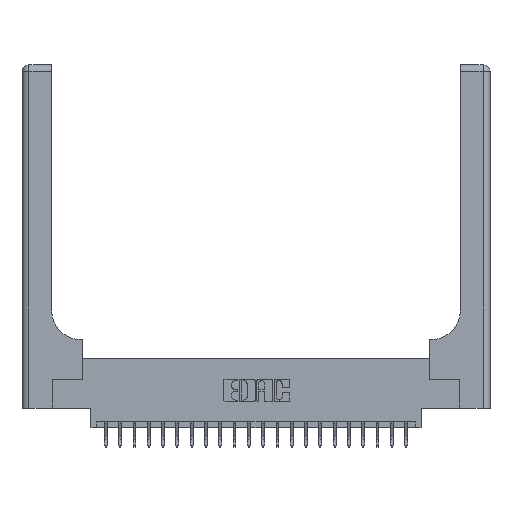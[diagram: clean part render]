
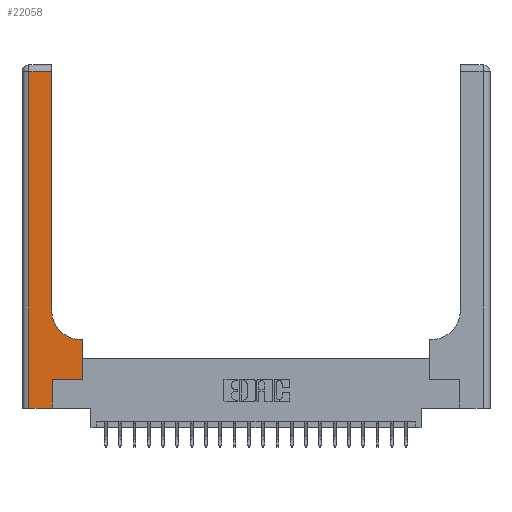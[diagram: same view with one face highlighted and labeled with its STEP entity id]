
A CAD part, top view. The second image highlights one B-rep face of the part: STEP entity #22058.
In plain terms, the highlighted planar face has unit normal (0, 0, 1).
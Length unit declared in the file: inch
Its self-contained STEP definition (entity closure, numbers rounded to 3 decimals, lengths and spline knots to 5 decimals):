
#354 = EDGE_CURVE ( 'NONE', #22687, #10060, #12485, .T. ) ;
#373 = DIRECTION ( 'NONE',  ( 0., 1., 0. ) ) ;
#702 = LINE ( 'NONE', #4646, #15385 ) ;
#1001 = VECTOR ( 'NONE', #373, 39.37008 ) ;
#1031 = VERTEX_POINT ( 'NONE', #20123 ) ;
#1869 = ORIENTED_EDGE ( 'NONE', *, *, #354, .T. ) ;
#2169 = FACE_OUTER_BOUND ( 'NONE', #19576, .T. ) ;
#2433 = AXIS2_PLACEMENT_3D ( 'NONE', #6753, #10251, #6408 ) ;
#2527 = CARTESIAN_POINT ( 'NONE',  ( 0.26, 0.85, 0.37 ) ) ;
#2699 = EDGE_CURVE ( 'NONE', #20403, #5717, #10989, .T. ) ;
#2760 = ORIENTED_EDGE ( 'NONE', *, *, #2699, .T. ) ;
#3105 = VECTOR ( 'NONE', #9244, 39.37008 ) ;
#3451 = DIRECTION ( 'NONE',  ( 0., 0., -1. ) ) ;
#3487 = CARTESIAN_POINT ( 'NONE',  ( 0.26, 0.6, 0.37 ) ) ;
#4061 = VERTEX_POINT ( 'NONE', #10677 ) ;
#4200 = VERTEX_POINT ( 'NONE', #21953 ) ;
#4477 = ORIENTED_EDGE ( 'NONE', *, *, #10024, .T. ) ;
#4501 = EDGE_CURVE ( 'NONE', #14902, #20403, #19275, .T. ) ;
#4569 = VERTEX_POINT ( 'NONE', #9562 ) ;
#4646 = CARTESIAN_POINT ( 'NONE',  ( 0.265, 0.25, 0.37 ) ) ;
#5717 = VERTEX_POINT ( 'NONE', #22329 ) ;
#5737 = AXIS2_PLACEMENT_3D ( 'NONE', #9171, #3451, #10915 ) ;
#6200 = ORIENTED_EDGE ( 'NONE', *, *, #15142, .T. ) ;
#6408 = DIRECTION ( 'NONE',  ( 1., 0., 0. ) ) ;
#6609 = CARTESIAN_POINT ( 'NONE',  ( 0.06, 0., 0.37 ) ) ;
#6746 = VECTOR ( 'NONE', #12349, 39.37008 ) ;
#6753 = CARTESIAN_POINT ( 'NONE',  ( 0.51, 0.85, 0.37 ) ) ;
#6793 = VECTOR ( 'NONE', #21531, 39.37008 ) ;
#6999 = CARTESIAN_POINT ( 'NONE',  ( 0., 2.94, 0.37 ) ) ;
#7068 = VECTOR ( 'NONE', #19384, 39.37008 ) ;
#7330 = LINE ( 'NONE', #14432, #6793 ) ;
#7454 = CARTESIAN_POINT ( 'NONE',  ( 0.265, 0., 0.37 ) ) ;
#7826 = DIRECTION ( 'NONE',  ( 1., 0., 0. ) ) ;
#7967 = CARTESIAN_POINT ( 'NONE',  ( 0.51, 0.6, 0.37 ) ) ;
#8855 = DIRECTION ( 'NONE',  ( -1., 0., 0. ) ) ;
#8887 = CARTESIAN_POINT ( 'NONE',  ( 0., 0., 0.37 ) ) ;
#9171 = CARTESIAN_POINT ( 'NONE',  ( 0., 3., 0.37 ) ) ;
#9244 = DIRECTION ( 'NONE',  ( 1., 0., 0. ) ) ;
#9562 = CARTESIAN_POINT ( 'NONE',  ( 0.26, 2.94, 0.37 ) ) ;
#10024 = EDGE_CURVE ( 'NONE', #4200, #1031, #7330, .T. ) ;
#10060 = VERTEX_POINT ( 'NONE', #2527 ) ;
#10251 = DIRECTION ( 'NONE',  ( 0., 0., -1. ) ) ;
#10677 = CARTESIAN_POINT ( 'NONE',  ( 0.265, 0.25, 0.37 ) ) ;
#10915 = DIRECTION ( 'NONE',  ( -1., 0., 0. ) ) ;
#10989 = LINE ( 'NONE', #8887, #3105 ) ;
#12276 = CARTESIAN_POINT ( 'NONE',  ( 0.06, 3., 0.37 ) ) ;
#12349 = DIRECTION ( 'NONE',  ( -1., 0., 0. ) ) ;
#12485 = CIRCLE ( 'NONE', #2433, 0.25 ) ;
#12688 = LINE ( 'NONE', #7454, #14801 ) ;
#13107 = ORIENTED_EDGE ( 'NONE', *, *, #4501, .T. ) ;
#13527 = ORIENTED_EDGE ( 'NONE', *, *, #17613, .T. ) ;
#14432 = CARTESIAN_POINT ( 'NONE',  ( 0.528, 0.25, 0.37 ) ) ;
#14550 = DIRECTION ( 'NONE',  ( 0., 1., 0. ) ) ;
#14801 = VECTOR ( 'NONE', #14550, 39.37008 ) ;
#14902 = VERTEX_POINT ( 'NONE', #15537 ) ;
#15142 = EDGE_CURVE ( 'NONE', #10060, #4569, #21587, .T. ) ;
#15158 = ORIENTED_EDGE ( 'NONE', *, *, #18719, .T. ) ;
#15178 = ORIENTED_EDGE ( 'NONE', *, *, #18808, .T. ) ;
#15301 = VECTOR ( 'NONE', #8855, 39.37008 ) ;
#15385 = VECTOR ( 'NONE', #7826, 39.37008 ) ;
#15537 = CARTESIAN_POINT ( 'NONE',  ( 0.06, 2.94, 0.37 ) ) ;
#16147 = PLANE ( 'NONE',  #5737 ) ;
#16344 = CARTESIAN_POINT ( 'NONE',  ( 0.26, 3., 0.37 ) ) ;
#17476 = LINE ( 'NONE', #3487, #15301 ) ;
#17613 = EDGE_CURVE ( 'NONE', #5717, #4061, #12688, .T. ) ;
#18719 = EDGE_CURVE ( 'NONE', #4569, #14902, #19348, .T. ) ;
#18808 = EDGE_CURVE ( 'NONE', #1031, #22687, #17476, .T. ) ;
#19275 = LINE ( 'NONE', #12276, #7068 ) ;
#19348 = LINE ( 'NONE', #6999, #6746 ) ;
#19384 = DIRECTION ( 'NONE',  ( 0., -1., 0. ) ) ;
#19576 = EDGE_LOOP ( 'NONE', ( #6200, #15158, #13107, #2760, #13527, #22527, #4477, #15178, #1869 ) ) ;
#20123 = CARTESIAN_POINT ( 'NONE',  ( 0.528, 0.6, 0.37 ) ) ;
#20403 = VERTEX_POINT ( 'NONE', #6609 ) ;
#21531 = DIRECTION ( 'NONE',  ( 0., 1., 0. ) ) ;
#21587 = LINE ( 'NONE', #16344, #1001 ) ;
#21614 = EDGE_CURVE ( 'NONE', #4061, #4200, #702, .T. ) ;
#21953 = CARTESIAN_POINT ( 'NONE',  ( 0.528, 0.25, 0.37 ) ) ;
#22058 = ADVANCED_FACE ( 'NONE', ( #2169 ), #16147, .F. ) ;
#22329 = CARTESIAN_POINT ( 'NONE',  ( 0.265, 0., 0.37 ) ) ;
#22527 = ORIENTED_EDGE ( 'NONE', *, *, #21614, .T. ) ;
#22687 = VERTEX_POINT ( 'NONE', #7967 ) ;
